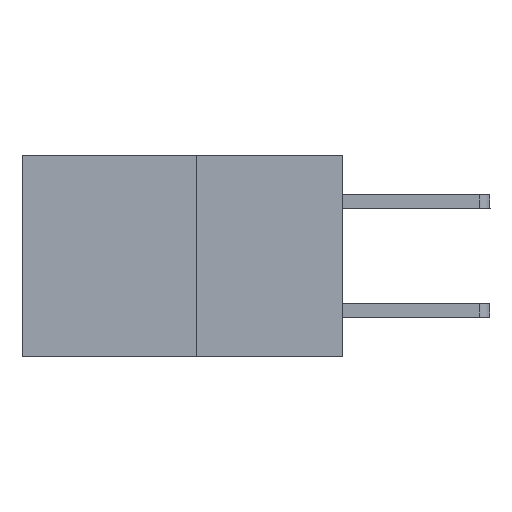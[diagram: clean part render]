
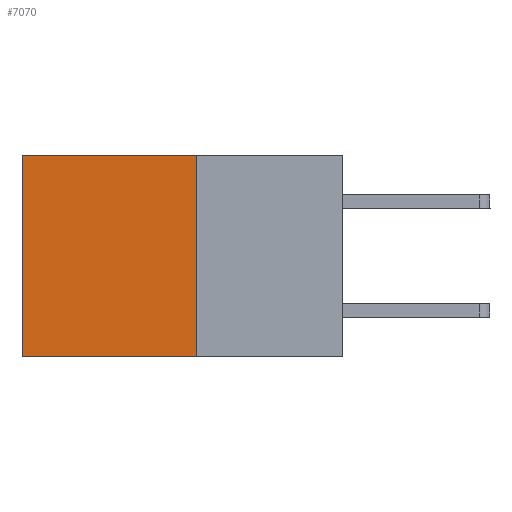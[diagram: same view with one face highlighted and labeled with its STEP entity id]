
A CAD part, left-side view. The second image highlights one B-rep face of the part: STEP entity #7070.
In plain terms, the highlighted planar face has unit normal (-1, 0, 0).
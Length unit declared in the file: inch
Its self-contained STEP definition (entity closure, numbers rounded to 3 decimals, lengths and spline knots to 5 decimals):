
#311 = ORIENTED_EDGE ( 'NONE', *, *, #612, .T. ) ;
#550 = EDGE_CURVE ( 'NONE', #3812, #3413, #9028, .T. ) ;
#612 = EDGE_CURVE ( 'NONE', #8554, #3812, #10852, .T. ) ;
#810 = CARTESIAN_POINT ( 'NONE',  ( 0.277, 0.27, 0. ) ) ;
#1136 = CARTESIAN_POINT ( 'NONE',  ( 0.277, 0.59, -0.37 ) ) ;
#1626 = EDGE_CURVE ( 'NONE', #8554, #10041, #9539, .T. ) ;
#2832 = VECTOR ( 'NONE', #4803, 39.37008 ) ;
#3023 = EDGE_LOOP ( 'NONE', ( #3850, #3484, #9167, #311 ) ) ;
#3234 = CARTESIAN_POINT ( 'NONE',  ( 0.277, 0.59, -0.37 ) ) ;
#3413 = VERTEX_POINT ( 'NONE', #3234 ) ;
#3484 = ORIENTED_EDGE ( 'NONE', *, *, #9899, .F. ) ;
#3689 = LINE ( 'NONE', #5096, #8220 ) ;
#3812 = VERTEX_POINT ( 'NONE', #4711 ) ;
#3850 = ORIENTED_EDGE ( 'NONE', *, *, #550, .T. ) ;
#3942 = FACE_OUTER_BOUND ( 'NONE', #3023, .T. ) ;
#4528 = VECTOR ( 'NONE', #4826, 39.37008 ) ;
#4711 = CARTESIAN_POINT ( 'NONE',  ( 0.277, 0.59, 0. ) ) ;
#4803 = DIRECTION ( 'NONE',  ( 0., 1., 0. ) ) ;
#4826 = DIRECTION ( 'NONE',  ( 0., 0., -1. ) ) ;
#5096 = CARTESIAN_POINT ( 'NONE',  ( 0.277, 0.27, -0.37 ) ) ;
#6077 = CARTESIAN_POINT ( 'NONE',  ( 0.277, 0.27, -0.37 ) ) ;
#6734 = AXIS2_PLACEMENT_3D ( 'NONE', #10549, #10535, #8947 ) ;
#7070 = ADVANCED_FACE ( 'NONE', ( #3942 ), #10588, .F. ) ;
#7313 = DIRECTION ( 'NONE',  ( 0., 0., -1. ) ) ;
#7570 = CARTESIAN_POINT ( 'NONE',  ( 0.277, 0.27, 0. ) ) ;
#8220 = VECTOR ( 'NONE', #10849, 39.37008 ) ;
#8417 = CARTESIAN_POINT ( 'NONE',  ( 0.277, 0.27, -0.37 ) ) ;
#8554 = VERTEX_POINT ( 'NONE', #7570 ) ;
#8947 = DIRECTION ( 'NONE',  ( 0., 0., -1. ) ) ;
#9001 = VECTOR ( 'NONE', #7313, 39.37008 ) ;
#9028 = LINE ( 'NONE', #1136, #4528 ) ;
#9167 = ORIENTED_EDGE ( 'NONE', *, *, #1626, .F. ) ;
#9539 = LINE ( 'NONE', #8417, #9001 ) ;
#9899 = EDGE_CURVE ( 'NONE', #10041, #3413, #3689, .T. ) ;
#10041 = VERTEX_POINT ( 'NONE', #6077 ) ;
#10535 = DIRECTION ( 'NONE',  ( 1., 0., 0. ) ) ;
#10549 = CARTESIAN_POINT ( 'NONE',  ( 0.277, 0.27, -0.37 ) ) ;
#10588 = PLANE ( 'NONE',  #6734 ) ;
#10849 = DIRECTION ( 'NONE',  ( 0., 1., 0. ) ) ;
#10852 = LINE ( 'NONE', #810, #2832 ) ;
